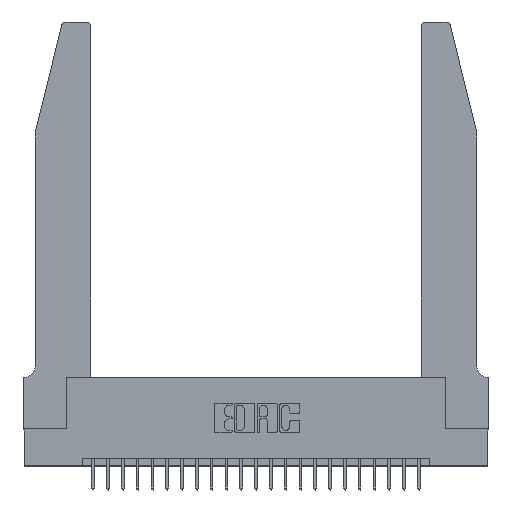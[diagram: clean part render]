
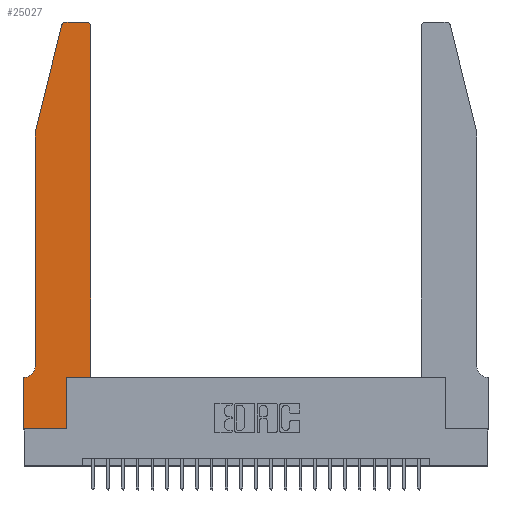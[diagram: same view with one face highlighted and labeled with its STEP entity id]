
A CAD part, top view. The second image highlights one B-rep face of the part: STEP entity #25027.
In plain terms, the highlighted planar face has unit normal (0, 0, 1).
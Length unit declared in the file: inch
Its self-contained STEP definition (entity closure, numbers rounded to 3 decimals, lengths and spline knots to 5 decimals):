
#287 = ORIENTED_EDGE ( 'NONE', *, *, #12474, .T. ) ;
#661 = VERTEX_POINT ( 'NONE', #16979 ) ;
#878 = DIRECTION ( 'NONE',  ( 1., 0., 0. ) ) ;
#903 = CARTESIAN_POINT ( 'NONE',  ( 0., 0., 0.37 ) ) ;
#1169 = LINE ( 'NONE', #17896, #16212 ) ;
#1232 = VERTEX_POINT ( 'NONE', #24202 ) ;
#1702 = VERTEX_POINT ( 'NONE', #10733 ) ;
#1707 = ORIENTED_EDGE ( 'NONE', *, *, #9136, .T. ) ;
#1781 = DIRECTION ( 'NONE',  ( 0., 1., 0. ) ) ;
#1905 = EDGE_LOOP ( 'NONE', ( #1707, #3994, #2524, #11149, #25004, #25408, #10683, #2104, #287, #12388, #6870, #11797 ) ) ;
#1915 = AXIS2_PLACEMENT_3D ( 'NONE', #6695, #20421, #8654 ) ;
#2104 = ORIENTED_EDGE ( 'NONE', *, *, #24167, .T. ) ;
#2298 = DIRECTION ( 'NONE',  ( 1., 0., 0. ) ) ;
#2524 = ORIENTED_EDGE ( 'NONE', *, *, #6262, .T. ) ;
#3293 = CARTESIAN_POINT ( 'NONE',  ( 0.4205, 2.75, 0.37 ) ) ;
#3430 = VECTOR ( 'NONE', #5915, 39.37008 ) ;
#3994 = ORIENTED_EDGE ( 'NONE', *, *, #13447, .T. ) ;
#5473 = DIRECTION ( 'NONE',  ( -1., 0., 0. ) ) ;
#5915 = DIRECTION ( 'NONE',  ( -0.239, -0.971, 0. ) ) ;
#5920 = CARTESIAN_POINT ( 'NONE',  ( 0., 0.35, 0.37 ) ) ;
#6262 = EDGE_CURVE ( 'NONE', #12025, #1702, #8631, .T. ) ;
#6322 = LINE ( 'NONE', #23121, #11515 ) ;
#6695 = CARTESIAN_POINT ( 'NONE',  ( 0.284, 2.72, 0.37 ) ) ;
#6809 = CARTESIAN_POINT ( 'NONE',  ( 0.0755, 2., 0.37 ) ) ;
#6870 = ORIENTED_EDGE ( 'NONE', *, *, #16081, .T. ) ;
#7869 = CARTESIAN_POINT ( 'NONE',  ( 0.2865, 0., 0.37 ) ) ;
#7940 = VERTEX_POINT ( 'NONE', #5920 ) ;
#8327 = VECTOR ( 'NONE', #10888, 39.37008 ) ;
#8631 = LINE ( 'NONE', #13705, #3430 ) ;
#8654 = DIRECTION ( 'NONE',  ( 1., 0., 0. ) ) ;
#9136 = EDGE_CURVE ( 'NONE', #23765, #12445, #6322, .T. ) ;
#9238 = VECTOR ( 'NONE', #1781, 39.37008 ) ;
#9743 = DIRECTION ( 'NONE',  ( 0., 1., 0. ) ) ;
#9811 = CARTESIAN_POINT ( 'NONE',  ( 0.0055, 0.35, 0.37 ) ) ;
#9912 = DIRECTION ( 'NONE',  ( 0., 0., 1. ) ) ;
#10603 = CARTESIAN_POINT ( 'NONE',  ( 0.2865, 0.35, 0.37 ) ) ;
#10607 = LINE ( 'NONE', #6809, #15838 ) ;
#10672 = PLANE ( 'NONE',  #20344 ) ;
#10683 = ORIENTED_EDGE ( 'NONE', *, *, #11596, .T. ) ;
#10733 = CARTESIAN_POINT ( 'NONE',  ( 0.0755, 2., 0.37 ) ) ;
#10751 = VERTEX_POINT ( 'NONE', #10603 ) ;
#10888 = DIRECTION ( 'NONE',  ( 0., -1., 0. ) ) ;
#11006 = EDGE_CURVE ( 'NONE', #19849, #16795, #20012, .T. ) ;
#11147 = FACE_OUTER_BOUND ( 'NONE', #1905, .T. ) ;
#11149 = ORIENTED_EDGE ( 'NONE', *, *, #23632, .T. ) ;
#11449 = CARTESIAN_POINT ( 'NONE',  ( 0.0055, 0.42, 0.37 ) ) ;
#11515 = VECTOR ( 'NONE', #5473, 39.37008 ) ;
#11596 = EDGE_CURVE ( 'NONE', #7940, #20177, #23365, .T. ) ;
#11797 = ORIENTED_EDGE ( 'NONE', *, *, #19097, .T. ) ;
#12025 = VERTEX_POINT ( 'NONE', #18064 ) ;
#12388 = ORIENTED_EDGE ( 'NONE', *, *, #21996, .T. ) ;
#12445 = VERTEX_POINT ( 'NONE', #17438 ) ;
#12474 = EDGE_CURVE ( 'NONE', #14283, #10751, #18083, .T. ) ;
#12633 = DIRECTION ( 'NONE',  ( -1., 0., 0. ) ) ;
#12637 = DIRECTION ( 'NONE',  ( 0., 0., 1. ) ) ;
#13224 = AXIS2_PLACEMENT_3D ( 'NONE', #11449, #25180, #13421 ) ;
#13421 = DIRECTION ( 'NONE',  ( -1., 0., 0. ) ) ;
#13447 = EDGE_CURVE ( 'NONE', #12445, #12025, #24493, .T. ) ;
#13705 = CARTESIAN_POINT ( 'NONE',  ( 0.0755, 2., 0.37 ) ) ;
#13952 = VECTOR ( 'NONE', #18086, 39.37008 ) ;
#14220 = CARTESIAN_POINT ( 'NONE',  ( 0., 0., 0.37 ) ) ;
#14283 = VERTEX_POINT ( 'NONE', #7869 ) ;
#15500 = CARTESIAN_POINT ( 'NONE',  ( 0.4505, 0.35, 0.37 ) ) ;
#15838 = VECTOR ( 'NONE', #20532, 39.37008 ) ;
#15892 = VECTOR ( 'NONE', #12633, 39.37008 ) ;
#15982 = AXIS2_PLACEMENT_3D ( 'NONE', #21662, #9912, #23624 ) ;
#16081 = EDGE_CURVE ( 'NONE', #661, #1232, #19669, .T. ) ;
#16212 = VECTOR ( 'NONE', #2298, 39.37008 ) ;
#16301 = CARTESIAN_POINT ( 'NONE',  ( 0.0755, 0.42, 0.37 ) ) ;
#16795 = VERTEX_POINT ( 'NONE', #9811 ) ;
#16979 = CARTESIAN_POINT ( 'NONE',  ( 0.4505, 0.35, 0.37 ) ) ;
#17438 = CARTESIAN_POINT ( 'NONE',  ( 0.284, 2.75, 0.37 ) ) ;
#17462 = VECTOR ( 'NONE', #9743, 39.37008 ) ;
#17599 = EDGE_CURVE ( 'NONE', #16795, #7940, #21125, .T. ) ;
#17896 = CARTESIAN_POINT ( 'NONE',  ( 0.4505, 0.35, 0.37 ) ) ;
#18064 = CARTESIAN_POINT ( 'NONE',  ( 0.25487, 2.72718, 0.37 ) ) ;
#18083 = LINE ( 'NONE', #19516, #17462 ) ;
#18086 = DIRECTION ( 'NONE',  ( 1., 0., 0. ) ) ;
#19097 = EDGE_CURVE ( 'NONE', #1232, #23765, #25032, .T. ) ;
#19516 = CARTESIAN_POINT ( 'NONE',  ( 0.2865, 0.35, 0.37 ) ) ;
#19669 = LINE ( 'NONE', #15500, #9238 ) ;
#19849 = VERTEX_POINT ( 'NONE', #16301 ) ;
#20012 = CIRCLE ( 'NONE', #13224, 0.07 ) ;
#20177 = VERTEX_POINT ( 'NONE', #903 ) ;
#20344 = AXIS2_PLACEMENT_3D ( 'NONE', #24320, #12637, #878 ) ;
#20421 = DIRECTION ( 'NONE',  ( 0., 0., 1. ) ) ;
#20472 = CARTESIAN_POINT ( 'NONE',  ( 0.0755, 0.35, 0.37 ) ) ;
#20532 = DIRECTION ( 'NONE',  ( 0., -1., 0. ) ) ;
#21125 = LINE ( 'NONE', #20472, #15892 ) ;
#21662 = CARTESIAN_POINT ( 'NONE',  ( 0.4205, 2.72, 0.37 ) ) ;
#21996 = EDGE_CURVE ( 'NONE', #10751, #661, #1169, .T. ) ;
#22640 = CARTESIAN_POINT ( 'NONE',  ( 0., 0., 0.37 ) ) ;
#23121 = CARTESIAN_POINT ( 'NONE',  ( 0.2605, 2.75, 0.37 ) ) ;
#23365 = LINE ( 'NONE', #22640, #8327 ) ;
#23624 = DIRECTION ( 'NONE',  ( 1., 0., 0. ) ) ;
#23632 = EDGE_CURVE ( 'NONE', #1702, #19849, #10607, .T. ) ;
#23765 = VERTEX_POINT ( 'NONE', #3293 ) ;
#24167 = EDGE_CURVE ( 'NONE', #20177, #14283, #25015, .T. ) ;
#24202 = CARTESIAN_POINT ( 'NONE',  ( 0.4505, 2.72, 0.37 ) ) ;
#24320 = CARTESIAN_POINT ( 'NONE',  ( 0., 0.35, 0.37 ) ) ;
#24493 = CIRCLE ( 'NONE', #1915, 0.03 ) ;
#25004 = ORIENTED_EDGE ( 'NONE', *, *, #11006, .T. ) ;
#25015 = LINE ( 'NONE', #14220, #13952 ) ;
#25027 = ADVANCED_FACE ( 'NONE', ( #11147 ), #10672, .T. ) ;
#25032 = CIRCLE ( 'NONE', #15982, 0.03 ) ;
#25180 = DIRECTION ( 'NONE',  ( 0., 0., -1. ) ) ;
#25408 = ORIENTED_EDGE ( 'NONE', *, *, #17599, .T. ) ;
